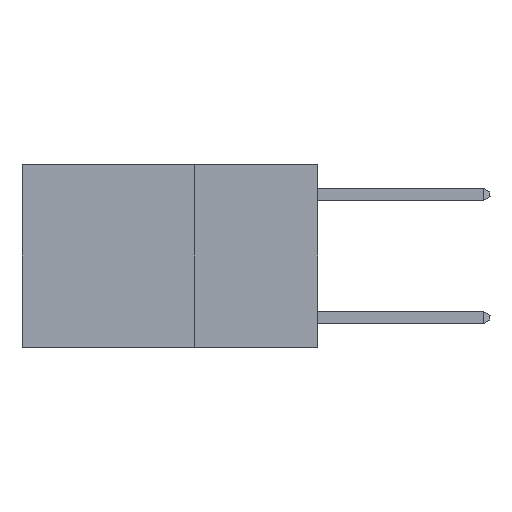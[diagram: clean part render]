
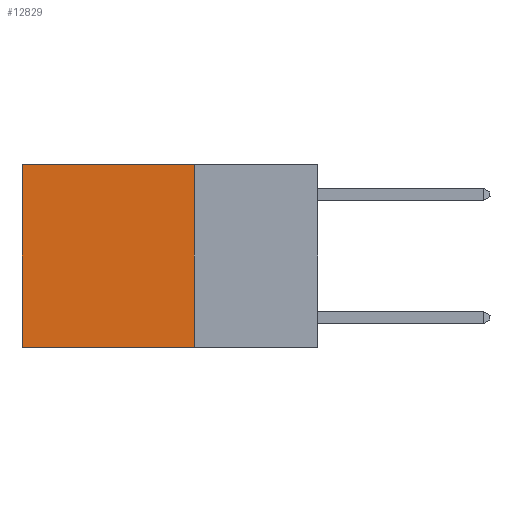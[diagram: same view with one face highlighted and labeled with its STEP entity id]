
A CAD part, left-side view. The second image highlights one B-rep face of the part: STEP entity #12829.
In plain terms, the highlighted planar face has unit normal (-1, 0, 0).
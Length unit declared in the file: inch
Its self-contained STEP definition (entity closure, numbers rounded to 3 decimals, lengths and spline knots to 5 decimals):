
#489 = CARTESIAN_POINT ( 'NONE',  ( 0.2625, 0.25, 0. ) ) ;
#3076 = VERTEX_POINT ( 'NONE', #11441 ) ;
#3913 = EDGE_CURVE ( 'NONE', #17972, #3076, #8107, .T. ) ;
#4780 = EDGE_CURVE ( 'NONE', #3076, #24903, #24247, .T. ) ;
#4781 = AXIS2_PLACEMENT_3D ( 'NONE', #9106, #14017, #4932 ) ;
#4932 = DIRECTION ( 'NONE',  ( 0., 0., -1. ) ) ;
#5009 = DIRECTION ( 'NONE',  ( 0., 0., -1. ) ) ;
#6849 = PLANE ( 'NONE',  #4781 ) ;
#7447 = DIRECTION ( 'NONE',  ( 0., 1., 0. ) ) ;
#8107 = LINE ( 'NONE', #19562, #23878 ) ;
#8666 = VECTOR ( 'NONE', #5009, 39.37008 ) ;
#9106 = CARTESIAN_POINT ( 'NONE',  ( 0.2625, 0.25, 0. ) ) ;
#10348 = ORIENTED_EDGE ( 'NONE', *, *, #3913, .T. ) ;
#11002 = ORIENTED_EDGE ( 'NONE', *, *, #24463, .F. ) ;
#11441 = CARTESIAN_POINT ( 'NONE',  ( 0.2625, 0.6, 0. ) ) ;
#12829 = ADVANCED_FACE ( 'NONE', ( #16378 ), #6849, .F. ) ;
#14017 = DIRECTION ( 'NONE',  ( 1., 0., 0. ) ) ;
#15277 = CARTESIAN_POINT ( 'NONE',  ( 0.2625, 0.6, 0. ) ) ;
#16378 = FACE_OUTER_BOUND ( 'NONE', #20316, .T. ) ;
#16409 = DIRECTION ( 'NONE',  ( 0., 0., -1. ) ) ;
#16944 = ORIENTED_EDGE ( 'NONE', *, *, #20091, .F. ) ;
#17972 = VERTEX_POINT ( 'NONE', #27674 ) ;
#18263 = VECTOR ( 'NONE', #16409, 39.37008 ) ;
#19372 = VERTEX_POINT ( 'NONE', #23041 ) ;
#19562 = CARTESIAN_POINT ( 'NONE',  ( 0.2625, 0.25, 0. ) ) ;
#20091 = EDGE_CURVE ( 'NONE', #17972, #19372, #25234, .T. ) ;
#20316 = EDGE_LOOP ( 'NONE', ( #26679, #11002, #16944, #10348 ) ) ;
#23041 = CARTESIAN_POINT ( 'NONE',  ( 0.2625, 0.25, -0.37 ) ) ;
#23042 = CARTESIAN_POINT ( 'NONE',  ( 0.2625, 0.6, -0.37 ) ) ;
#23234 = LINE ( 'NONE', #25780, #26011 ) ;
#23878 = VECTOR ( 'NONE', #26589, 39.37008 ) ;
#24247 = LINE ( 'NONE', #15277, #8666 ) ;
#24463 = EDGE_CURVE ( 'NONE', #19372, #24903, #23234, .T. ) ;
#24903 = VERTEX_POINT ( 'NONE', #23042 ) ;
#25234 = LINE ( 'NONE', #489, #18263 ) ;
#25780 = CARTESIAN_POINT ( 'NONE',  ( 0.2625, 0.25, -0.37 ) ) ;
#26011 = VECTOR ( 'NONE', #7447, 39.37008 ) ;
#26589 = DIRECTION ( 'NONE',  ( 0., 1., 0. ) ) ;
#26679 = ORIENTED_EDGE ( 'NONE', *, *, #4780, .T. ) ;
#27674 = CARTESIAN_POINT ( 'NONE',  ( 0.2625, 0.25, 0. ) ) ;
